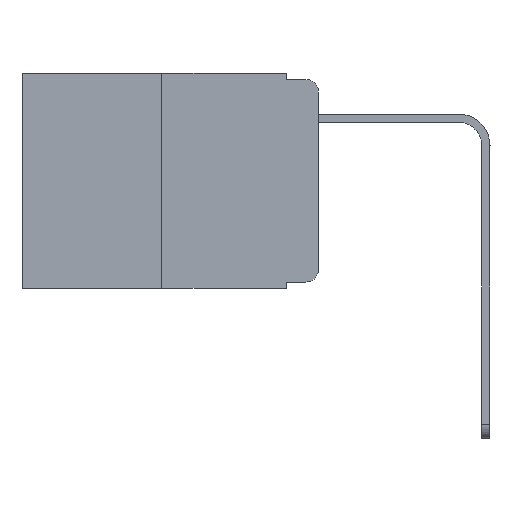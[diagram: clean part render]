
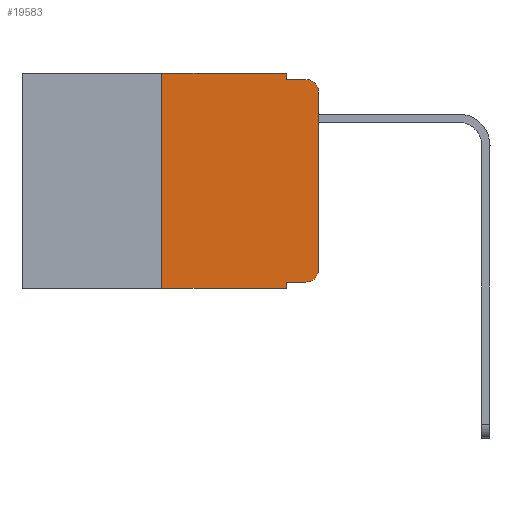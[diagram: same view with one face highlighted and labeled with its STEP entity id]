
A CAD part, left-side view. The second image highlights one B-rep face of the part: STEP entity #19583.
In plain terms, the highlighted planar face has unit normal (-1, 0, 0).
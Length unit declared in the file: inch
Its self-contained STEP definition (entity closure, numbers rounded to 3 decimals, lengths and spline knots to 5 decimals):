
#526 = VECTOR ( 'NONE', #13587, 39.37008 ) ;
#776 = VERTEX_POINT ( 'NONE', #14934 ) ;
#794 = CARTESIAN_POINT ( 'NONE',  ( 0., 0.051, -0.333 ) ) ;
#883 = CARTESIAN_POINT ( 'NONE',  ( 0., 0.051, -0.01 ) ) ;
#1001 = CARTESIAN_POINT ( 'NONE',  ( 0., 0.473, -0.343 ) ) ;
#1466 = EDGE_CURVE ( 'NONE', #10207, #9629, #7822, .T. ) ;
#2118 = CARTESIAN_POINT ( 'NONE',  ( 0., 0.473, 0. ) ) ;
#2518 = EDGE_CURVE ( 'NONE', #7171, #10806, #16251, .T. ) ;
#3116 = CARTESIAN_POINT ( 'NONE',  ( 0., 0.051, 0. ) ) ;
#3401 = ORIENTED_EDGE ( 'NONE', *, *, #23762, .T. ) ;
#3465 = CARTESIAN_POINT ( 'NONE',  ( 0., 0., 0. ) ) ;
#3749 = ORIENTED_EDGE ( 'NONE', *, *, #23065, .T. ) ;
#3833 = DIRECTION ( 'NONE',  ( 1., 0., 0. ) ) ;
#4029 = VECTOR ( 'NONE', #5167, 39.37008 ) ;
#4583 = LINE ( 'NONE', #19065, #526 ) ;
#4701 = CARTESIAN_POINT ( 'NONE',  ( 0., 0.051, -0.01 ) ) ;
#4706 = ORIENTED_EDGE ( 'NONE', *, *, #1466, .F. ) ;
#4829 = VERTEX_POINT ( 'NONE', #14426 ) ;
#4899 = VECTOR ( 'NONE', #15473, 39.37008 ) ;
#5167 = DIRECTION ( 'NONE',  ( 0., 0., 1. ) ) ;
#6070 = ORIENTED_EDGE ( 'NONE', *, *, #20120, .F. ) ;
#6574 = DIRECTION ( 'NONE',  ( 0., -1., 0. ) ) ;
#7171 = VERTEX_POINT ( 'NONE', #11416 ) ;
#7510 = LINE ( 'NONE', #19561, #9265 ) ;
#7571 = CARTESIAN_POINT ( 'NONE',  ( 0., 0.051, -0.333 ) ) ;
#7788 = FACE_OUTER_BOUND ( 'NONE', #14143, .T. ) ;
#7822 = LINE ( 'NONE', #4701, #11001 ) ;
#8520 = CARTESIAN_POINT ( 'NONE',  ( 0., 0.02, -0.313 ) ) ;
#8639 = VECTOR ( 'NONE', #10595, 39.37008 ) ;
#8947 = EDGE_CURVE ( 'NONE', #15241, #4829, #4583, .T. ) ;
#9265 = VECTOR ( 'NONE', #17677, 39.37008 ) ;
#9286 = PLANE ( 'NONE',  #14334 ) ;
#9629 = VERTEX_POINT ( 'NONE', #19437 ) ;
#9755 = DIRECTION ( 'NONE',  ( 0., -1., 0. ) ) ;
#10207 = VERTEX_POINT ( 'NONE', #883 ) ;
#10211 = CIRCLE ( 'NONE', #19359, 0.02 ) ;
#10531 = LINE ( 'NONE', #3116, #19281 ) ;
#10595 = DIRECTION ( 'NONE',  ( 0., -1., 0. ) ) ;
#10678 = CARTESIAN_POINT ( 'NONE',  ( 0., 0.473, 0. ) ) ;
#10806 = VERTEX_POINT ( 'NONE', #13826 ) ;
#11001 = VECTOR ( 'NONE', #6574, 39.37008 ) ;
#11133 = ORIENTED_EDGE ( 'NONE', *, *, #13544, .T. ) ;
#11416 = CARTESIAN_POINT ( 'NONE',  ( 0., 0., -0.313 ) ) ;
#11801 = ORIENTED_EDGE ( 'NONE', *, *, #19199, .F. ) ;
#12076 = ORIENTED_EDGE ( 'NONE', *, *, #8947, .F. ) ;
#12242 = DIRECTION ( 'NONE',  ( 0., 0., -1. ) ) ;
#12768 = VECTOR ( 'NONE', #9755, 39.37008 ) ;
#12926 = ORIENTED_EDGE ( 'NONE', *, *, #22482, .F. ) ;
#13013 = DIRECTION ( 'NONE',  ( 0., 0., -1. ) ) ;
#13544 = EDGE_CURVE ( 'NONE', #15241, #17822, #21193, .T. ) ;
#13561 = LINE ( 'NONE', #10678, #8639 ) ;
#13587 = DIRECTION ( 'NONE',  ( 0., 0., 1. ) ) ;
#13731 = CARTESIAN_POINT ( 'NONE',  ( 0., 0.02, -0.03 ) ) ;
#13826 = CARTESIAN_POINT ( 'NONE',  ( 0., 0., -0.03 ) ) ;
#14143 = EDGE_LOOP ( 'NONE', ( #16706, #3749, #4706, #11801, #6070, #12076, #11133, #12926, #22936, #3401 ) ) ;
#14334 = AXIS2_PLACEMENT_3D ( 'NONE', #2118, #3833, #13013 ) ;
#14426 = CARTESIAN_POINT ( 'NONE',  ( 0., 0.25, 0. ) ) ;
#14785 = CARTESIAN_POINT ( 'NONE',  ( 0., 0.25, -0.343 ) ) ;
#14934 = CARTESIAN_POINT ( 'NONE',  ( 0., 0.051, 0. ) ) ;
#15241 = VERTEX_POINT ( 'NONE', #14785 ) ;
#15416 = CIRCLE ( 'NONE', #19550, 0.02 ) ;
#15473 = DIRECTION ( 'NONE',  ( 0., -1., 0. ) ) ;
#15666 = DIRECTION ( 'NONE',  ( -1., 0., 0. ) ) ;
#16251 = LINE ( 'NONE', #3465, #4029 ) ;
#16349 = VERTEX_POINT ( 'NONE', #7571 ) ;
#16706 = ORIENTED_EDGE ( 'NONE', *, *, #2518, .T. ) ;
#17146 = VERTEX_POINT ( 'NONE', #22228 ) ;
#17677 = DIRECTION ( 'NONE',  ( 0., 0., -1. ) ) ;
#17822 = VERTEX_POINT ( 'NONE', #18242 ) ;
#18066 = DIRECTION ( 'NONE',  ( 0., 0., -1. ) ) ;
#18242 = CARTESIAN_POINT ( 'NONE',  ( 0., 0.051, -0.343 ) ) ;
#19065 = CARTESIAN_POINT ( 'NONE',  ( 0., 0.25, 0. ) ) ;
#19199 = EDGE_CURVE ( 'NONE', #776, #10207, #7510, .T. ) ;
#19232 = EDGE_CURVE ( 'NONE', #16349, #17146, #23180, .T. ) ;
#19281 = VECTOR ( 'NONE', #18066, 39.37008 ) ;
#19359 = AXIS2_PLACEMENT_3D ( 'NONE', #13731, #23227, #19446 ) ;
#19437 = CARTESIAN_POINT ( 'NONE',  ( 0., 0.02, -0.01 ) ) ;
#19446 = DIRECTION ( 'NONE',  ( 0., 0., -1. ) ) ;
#19550 = AXIS2_PLACEMENT_3D ( 'NONE', #8520, #15666, #12242 ) ;
#19561 = CARTESIAN_POINT ( 'NONE',  ( 0., 0.051, 0. ) ) ;
#19583 = ADVANCED_FACE ( 'NONE', ( #7788 ), #9286, .F. ) ;
#20120 = EDGE_CURVE ( 'NONE', #4829, #776, #13561, .T. ) ;
#21193 = LINE ( 'NONE', #1001, #12768 ) ;
#22228 = CARTESIAN_POINT ( 'NONE',  ( 0., 0.02, -0.333 ) ) ;
#22482 = EDGE_CURVE ( 'NONE', #16349, #17822, #10531, .T. ) ;
#22936 = ORIENTED_EDGE ( 'NONE', *, *, #19232, .T. ) ;
#23065 = EDGE_CURVE ( 'NONE', #10806, #9629, #10211, .T. ) ;
#23180 = LINE ( 'NONE', #794, #4899 ) ;
#23227 = DIRECTION ( 'NONE',  ( -1., 0., 0. ) ) ;
#23762 = EDGE_CURVE ( 'NONE', #17146, #7171, #15416, .T. ) ;
